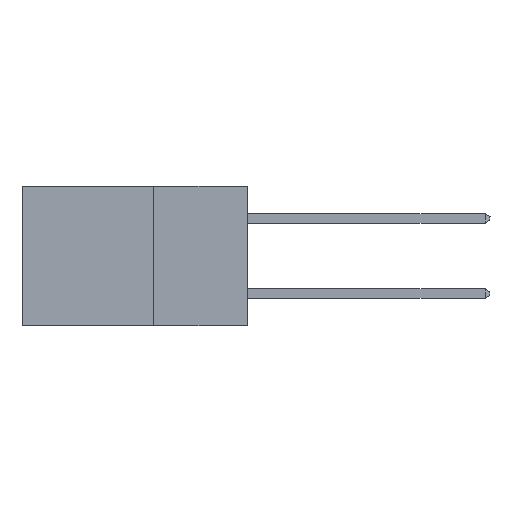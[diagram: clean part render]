
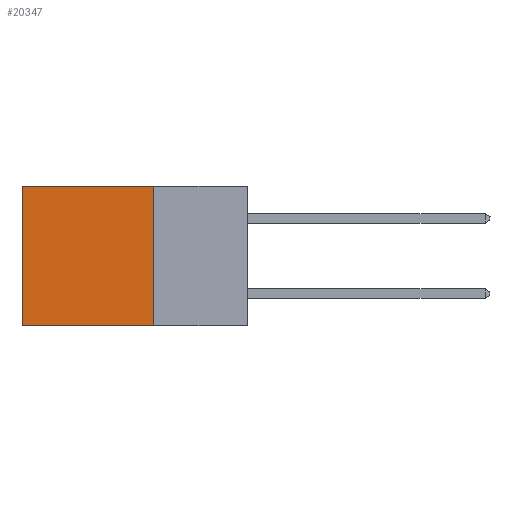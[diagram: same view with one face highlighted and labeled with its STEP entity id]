
A CAD part, left-side view. The second image highlights one B-rep face of the part: STEP entity #20347.
In plain terms, the highlighted planar face has unit normal (-1, 0, 0).
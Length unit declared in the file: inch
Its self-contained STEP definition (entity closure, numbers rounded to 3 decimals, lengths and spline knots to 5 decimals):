
#98 = CARTESIAN_POINT ( 'NONE',  ( 0.2615, 0.6, -0.37 ) ) ;
#682 = VECTOR ( 'NONE', #20884, 39.37008 ) ;
#1443 = VERTEX_POINT ( 'NONE', #8364 ) ;
#1933 = DIRECTION ( 'NONE',  ( 0., 1., 0. ) ) ;
#3066 = ORIENTED_EDGE ( 'NONE', *, *, #6603, .F. ) ;
#3387 = DIRECTION ( 'NONE',  ( 0., 0., -1. ) ) ;
#5002 = AXIS2_PLACEMENT_3D ( 'NONE', #5415, #14292, #12548 ) ;
#5382 = LINE ( 'NONE', #98, #11129 ) ;
#5415 = CARTESIAN_POINT ( 'NONE',  ( 0.2615, 0.25, -0.37 ) ) ;
#6026 = CARTESIAN_POINT ( 'NONE',  ( 0.2615, 0.6, -0.37 ) ) ;
#6603 = EDGE_CURVE ( 'NONE', #14281, #7947, #10948, .T. ) ;
#6727 = LINE ( 'NONE', #10591, #12547 ) ;
#7149 = PLANE ( 'NONE',  #5002 ) ;
#7462 = VECTOR ( 'NONE', #1933, 39.37008 ) ;
#7637 = EDGE_CURVE ( 'NONE', #13073, #14281, #8615, .T. ) ;
#7947 = VERTEX_POINT ( 'NONE', #6026 ) ;
#8364 = CARTESIAN_POINT ( 'NONE',  ( 0.2615, 0.6, 0. ) ) ;
#8615 = LINE ( 'NONE', #12248, #682 ) ;
#10591 = CARTESIAN_POINT ( 'NONE',  ( 0.2615, 0.25, 0. ) ) ;
#10948 = LINE ( 'NONE', #17976, #7462 ) ;
#10991 = EDGE_LOOP ( 'NONE', ( #18361, #3066, #20163, #17711 ) ) ;
#11129 = VECTOR ( 'NONE', #3387, 39.37008 ) ;
#12248 = CARTESIAN_POINT ( 'NONE',  ( 0.2615, 0.25, -0.37 ) ) ;
#12547 = VECTOR ( 'NONE', #15762, 39.37008 ) ;
#12548 = DIRECTION ( 'NONE',  ( 0., 0., -1. ) ) ;
#12617 = EDGE_CURVE ( 'NONE', #1443, #7947, #5382, .T. ) ;
#13073 = VERTEX_POINT ( 'NONE', #19940 ) ;
#14281 = VERTEX_POINT ( 'NONE', #15519 ) ;
#14292 = DIRECTION ( 'NONE',  ( 1., 0., 0. ) ) ;
#15519 = CARTESIAN_POINT ( 'NONE',  ( 0.2615, 0.25, -0.37 ) ) ;
#15762 = DIRECTION ( 'NONE',  ( 0., 1., 0. ) ) ;
#17711 = ORIENTED_EDGE ( 'NONE', *, *, #22584, .T. ) ;
#17814 = FACE_OUTER_BOUND ( 'NONE', #10991, .T. ) ;
#17976 = CARTESIAN_POINT ( 'NONE',  ( 0.2615, 0.25, -0.37 ) ) ;
#18361 = ORIENTED_EDGE ( 'NONE', *, *, #12617, .T. ) ;
#19940 = CARTESIAN_POINT ( 'NONE',  ( 0.2615, 0.25, 0. ) ) ;
#20163 = ORIENTED_EDGE ( 'NONE', *, *, #7637, .F. ) ;
#20347 = ADVANCED_FACE ( 'NONE', ( #17814 ), #7149, .F. ) ;
#20884 = DIRECTION ( 'NONE',  ( 0., 0., -1. ) ) ;
#22584 = EDGE_CURVE ( 'NONE', #13073, #1443, #6727, .T. ) ;
